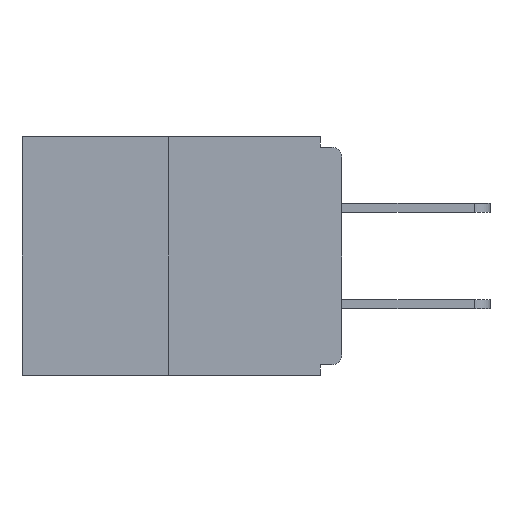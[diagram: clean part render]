
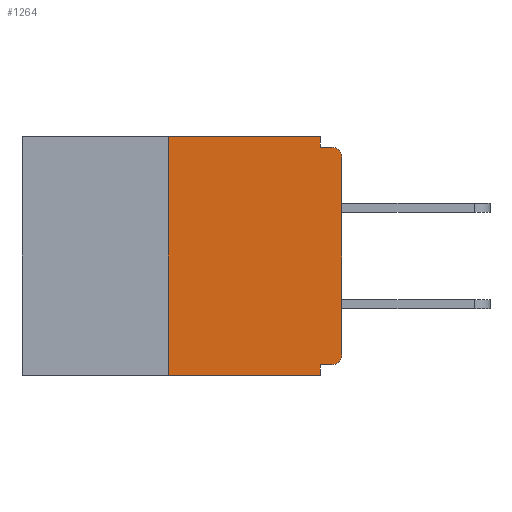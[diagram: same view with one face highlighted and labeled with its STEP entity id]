
A CAD part, left-side view. The second image highlights one B-rep face of the part: STEP entity #1264.
In plain terms, the highlighted planar face has unit normal (-1, 0, 0).
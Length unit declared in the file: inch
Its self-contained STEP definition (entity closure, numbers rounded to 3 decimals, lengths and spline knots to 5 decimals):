
#13 = VERTEX_POINT ( 'NONE', #9098 ) ;
#70 = PLANE ( 'NONE',  #7483 ) ;
#106 = CARTESIAN_POINT ( 'NONE',  ( 0., 0., -0.313 ) ) ;
#233 = CARTESIAN_POINT ( 'NONE',  ( 0., 0.015, -0.328 ) ) ;
#257 = VERTEX_POINT ( 'NONE', #3713 ) ;
#258 = VECTOR ( 'NONE', #2016, 39.37008 ) ;
#301 = VECTOR ( 'NONE', #2928, 39.37008 ) ;
#437 = CARTESIAN_POINT ( 'NONE',  ( 0., 0.015, -0.313 ) ) ;
#467 = EDGE_CURVE ( 'NONE', #257, #7925, #6603, .T. ) ;
#491 = LINE ( 'NONE', #2039, #7103 ) ;
#530 = LINE ( 'NONE', #6194, #5625 ) ;
#657 = DIRECTION ( 'NONE',  ( 0., 0., -1. ) ) ;
#773 = EDGE_LOOP ( 'NONE', ( #5973, #7715, #6632, #8573, #3966, #10042, #2218, #4634, #3448, #1753 ) ) ;
#827 = AXIS2_PLACEMENT_3D ( 'NONE', #437, #7068, #10386 ) ;
#1120 = FACE_OUTER_BOUND ( 'NONE', #773, .T. ) ;
#1135 = CARTESIAN_POINT ( 'NONE',  ( 0., 0., 0. ) ) ;
#1178 = VECTOR ( 'NONE', #657, 39.37008 ) ;
#1264 = ADVANCED_FACE ( 'NONE', ( #1120 ), #70, .F. ) ;
#1753 = ORIENTED_EDGE ( 'NONE', *, *, #9435, .F. ) ;
#1914 = CARTESIAN_POINT ( 'NONE',  ( 0., 0.031, -0.328 ) ) ;
#1928 = DIRECTION ( 'NONE',  ( 0., -1., 0. ) ) ;
#2016 = DIRECTION ( 'NONE',  ( 0., 0., 1. ) ) ;
#2039 = CARTESIAN_POINT ( 'NONE',  ( 0., 0.46, 0. ) ) ;
#2121 = CARTESIAN_POINT ( 'NONE',  ( 0., 0., -0.015 ) ) ;
#2218 = ORIENTED_EDGE ( 'NONE', *, *, #9771, .T. ) ;
#2260 = CARTESIAN_POINT ( 'NONE',  ( 0., 0.25, 0. ) ) ;
#2497 = VERTEX_POINT ( 'NONE', #1914 ) ;
#2506 = CARTESIAN_POINT ( 'NONE',  ( 0., 0.46, 0. ) ) ;
#2604 = DIRECTION ( 'NONE',  ( 0., 0., -1. ) ) ;
#2658 = EDGE_CURVE ( 'NONE', #13, #7925, #8629, .T. ) ;
#2784 = VECTOR ( 'NONE', #6239, 39.37008 ) ;
#2806 = DIRECTION ( 'NONE',  ( 0., -1., 0. ) ) ;
#2928 = DIRECTION ( 'NONE',  ( 0., -1., 0. ) ) ;
#3109 = EDGE_CURVE ( 'NONE', #6009, #3312, #10428, .T. ) ;
#3176 = EDGE_CURVE ( 'NONE', #7768, #5010, #6675, .T. ) ;
#3301 = DIRECTION ( 'NONE',  ( 0., 0., -1. ) ) ;
#3312 = VERTEX_POINT ( 'NONE', #2260 ) ;
#3392 = VECTOR ( 'NONE', #6133, 39.37008 ) ;
#3448 = ORIENTED_EDGE ( 'NONE', *, *, #2658, .F. ) ;
#3557 = CARTESIAN_POINT ( 'NONE',  ( 0., 0.031, -0.343 ) ) ;
#3615 = EDGE_CURVE ( 'NONE', #6009, #8756, #530, .T. ) ;
#3713 = CARTESIAN_POINT ( 'NONE',  ( 0., 0., -0.03 ) ) ;
#3935 = CARTESIAN_POINT ( 'NONE',  ( 0., 0.031, 0. ) ) ;
#3966 = ORIENTED_EDGE ( 'NONE', *, *, #7112, .F. ) ;
#4172 = EDGE_CURVE ( 'NONE', #2497, #8756, #4819, .T. ) ;
#4372 = CARTESIAN_POINT ( 'NONE',  ( 0., 0.031, -0.343 ) ) ;
#4400 = CARTESIAN_POINT ( 'NONE',  ( 0., 0., -0.328 ) ) ;
#4484 = CARTESIAN_POINT ( 'NONE',  ( 0., 0.25, 0. ) ) ;
#4560 = LINE ( 'NONE', #3935, #1178 ) ;
#4634 = ORIENTED_EDGE ( 'NONE', *, *, #467, .T. ) ;
#4819 = LINE ( 'NONE', #4372, #3392 ) ;
#5010 = VERTEX_POINT ( 'NONE', #106 ) ;
#5412 = VECTOR ( 'NONE', #8619, 39.37008 ) ;
#5625 = VECTOR ( 'NONE', #1928, 39.37008 ) ;
#5858 = DIRECTION ( 'NONE',  ( -1., 0., 0. ) ) ;
#5973 = ORIENTED_EDGE ( 'NONE', *, *, #10389, .F. ) ;
#6009 = VERTEX_POINT ( 'NONE', #7838 ) ;
#6133 = DIRECTION ( 'NONE',  ( 0., 0., -1. ) ) ;
#6194 = CARTESIAN_POINT ( 'NONE',  ( 0., 0.46, -0.343 ) ) ;
#6239 = DIRECTION ( 'NONE',  ( 0., 0., 1. ) ) ;
#6603 = CIRCLE ( 'NONE', #9739, 0.015 ) ;
#6632 = ORIENTED_EDGE ( 'NONE', *, *, #3615, .T. ) ;
#6675 = CIRCLE ( 'NONE', #827, 0.015 ) ;
#6783 = VERTEX_POINT ( 'NONE', #8809 ) ;
#7068 = DIRECTION ( 'NONE',  ( -1., 0., 0. ) ) ;
#7103 = VECTOR ( 'NONE', #2806, 39.37008 ) ;
#7112 = EDGE_CURVE ( 'NONE', #7768, #2497, #9807, .T. ) ;
#7483 = AXIS2_PLACEMENT_3D ( 'NONE', #2506, #8369, #2604 ) ;
#7715 = ORIENTED_EDGE ( 'NONE', *, *, #3109, .F. ) ;
#7768 = VERTEX_POINT ( 'NONE', #233 ) ;
#7838 = CARTESIAN_POINT ( 'NONE',  ( 0., 0.25, -0.343 ) ) ;
#7925 = VERTEX_POINT ( 'NONE', #8249 ) ;
#8249 = CARTESIAN_POINT ( 'NONE',  ( 0., 0.015, -0.015 ) ) ;
#8369 = DIRECTION ( 'NONE',  ( 1., 0., 0. ) ) ;
#8573 = ORIENTED_EDGE ( 'NONE', *, *, #4172, .F. ) ;
#8619 = DIRECTION ( 'NONE',  ( 0., 1., 0. ) ) ;
#8629 = LINE ( 'NONE', #2121, #301 ) ;
#8756 = VERTEX_POINT ( 'NONE', #3557 ) ;
#8809 = CARTESIAN_POINT ( 'NONE',  ( 0., 0.031, 0. ) ) ;
#9098 = CARTESIAN_POINT ( 'NONE',  ( 0., 0.031, -0.015 ) ) ;
#9435 = EDGE_CURVE ( 'NONE', #6783, #13, #4560, .T. ) ;
#9739 = AXIS2_PLACEMENT_3D ( 'NONE', #9945, #5858, #3301 ) ;
#9771 = EDGE_CURVE ( 'NONE', #5010, #257, #10160, .T. ) ;
#9807 = LINE ( 'NONE', #4400, #5412 ) ;
#9945 = CARTESIAN_POINT ( 'NONE',  ( 0., 0.015, -0.03 ) ) ;
#10042 = ORIENTED_EDGE ( 'NONE', *, *, #3176, .T. ) ;
#10160 = LINE ( 'NONE', #1135, #258 ) ;
#10386 = DIRECTION ( 'NONE',  ( 0., 0., -1. ) ) ;
#10389 = EDGE_CURVE ( 'NONE', #3312, #6783, #491, .T. ) ;
#10428 = LINE ( 'NONE', #4484, #2784 ) ;
